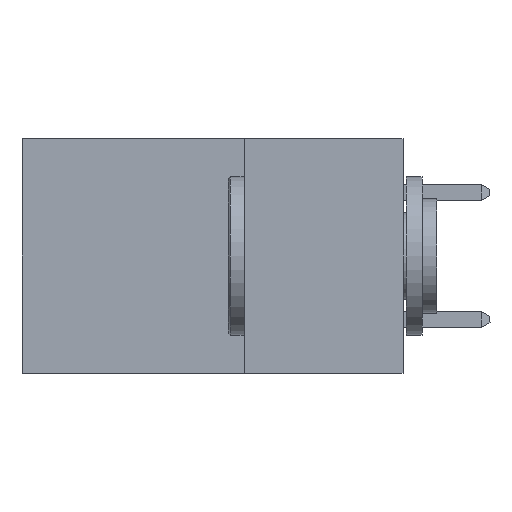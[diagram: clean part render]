
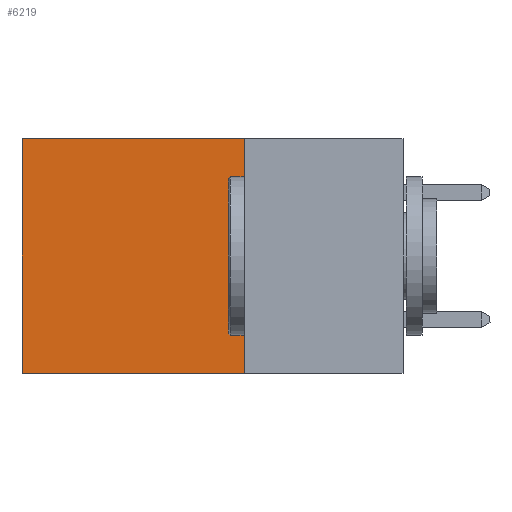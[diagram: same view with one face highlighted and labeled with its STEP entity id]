
A CAD part, left-side view. The second image highlights one B-rep face of the part: STEP entity #6219.
In plain terms, the highlighted planar face has unit normal (-1, 0, 0).
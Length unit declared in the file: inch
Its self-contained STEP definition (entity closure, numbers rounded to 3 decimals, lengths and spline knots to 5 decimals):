
#499 = EDGE_CURVE ( 'NONE', #13171, #10594, #16141, .T. ) ;
#581 = DIRECTION ( 'NONE',  ( 0., 1., 0. ) ) ;
#908 = EDGE_CURVE ( 'NONE', #18788, #4188, #7531, .T. ) ;
#1050 = DIRECTION ( 'NONE',  ( 0., 0., -1. ) ) ;
#1568 = EDGE_CURVE ( 'NONE', #18788, #13171, #19093, .T. ) ;
#1832 = ORIENTED_EDGE ( 'NONE', *, *, #499, .T. ) ;
#2378 = DIRECTION ( 'NONE',  ( 1., 0., 0. ) ) ;
#2687 = CARTESIAN_POINT ( 'NONE',  ( 0.2875, 0.25, 0. ) ) ;
#3364 = LINE ( 'NONE', #6845, #10744 ) ;
#3379 = VECTOR ( 'NONE', #1050, 39.37008 ) ;
#3401 = VECTOR ( 'NONE', #4257, 39.37008 ) ;
#4188 = VERTEX_POINT ( 'NONE', #17947 ) ;
#4257 = DIRECTION ( 'NONE',  ( 0., 0., -1. ) ) ;
#4541 = EDGE_LOOP ( 'NONE', ( #1832, #11898, #8236, #16576 ) ) ;
#6219 = ADVANCED_FACE ( 'NONE', ( #19917 ), #7020, .F. ) ;
#6595 = AXIS2_PLACEMENT_3D ( 'NONE', #11821, #2378, #13460 ) ;
#6845 = CARTESIAN_POINT ( 'NONE',  ( 0.2875, 0.25, -0.37 ) ) ;
#7020 = PLANE ( 'NONE',  #6595 ) ;
#7531 = LINE ( 'NONE', #2687, #3379 ) ;
#8044 = CARTESIAN_POINT ( 'NONE',  ( 0.2875, 0.6, -0.37 ) ) ;
#8236 = ORIENTED_EDGE ( 'NONE', *, *, #908, .F. ) ;
#10008 = DIRECTION ( 'NONE',  ( 0., 1., 0. ) ) ;
#10083 = CARTESIAN_POINT ( 'NONE',  ( 0.2875, 0.25, 0. ) ) ;
#10087 = EDGE_CURVE ( 'NONE', #4188, #10594, #3364, .T. ) ;
#10594 = VERTEX_POINT ( 'NONE', #8044 ) ;
#10744 = VECTOR ( 'NONE', #581, 39.37008 ) ;
#11821 = CARTESIAN_POINT ( 'NONE',  ( 0.2875, 0.25, 0. ) ) ;
#11898 = ORIENTED_EDGE ( 'NONE', *, *, #10087, .F. ) ;
#12600 = CARTESIAN_POINT ( 'NONE',  ( 0.2875, 0.6, 0. ) ) ;
#13171 = VERTEX_POINT ( 'NONE', #12600 ) ;
#13460 = DIRECTION ( 'NONE',  ( 0., 0., -1. ) ) ;
#14802 = VECTOR ( 'NONE', #10008, 39.37008 ) ;
#16141 = LINE ( 'NONE', #18309, #3401 ) ;
#16576 = ORIENTED_EDGE ( 'NONE', *, *, #1568, .T. ) ;
#17546 = CARTESIAN_POINT ( 'NONE',  ( 0.2875, 0.25, 0. ) ) ;
#17947 = CARTESIAN_POINT ( 'NONE',  ( 0.2875, 0.25, -0.37 ) ) ;
#18309 = CARTESIAN_POINT ( 'NONE',  ( 0.2875, 0.6, 0. ) ) ;
#18788 = VERTEX_POINT ( 'NONE', #17546 ) ;
#19093 = LINE ( 'NONE', #10083, #14802 ) ;
#19917 = FACE_OUTER_BOUND ( 'NONE', #4541, .T. ) ;
